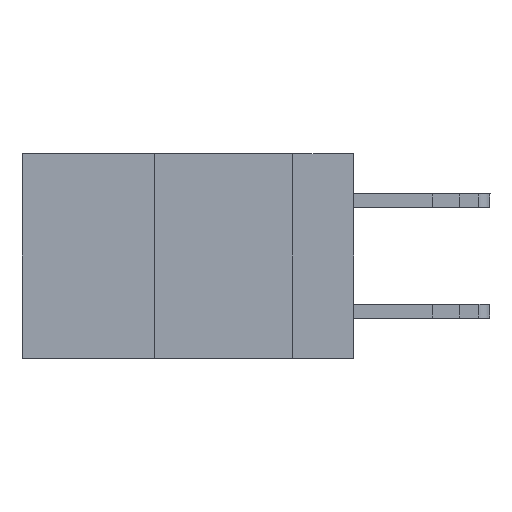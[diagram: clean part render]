
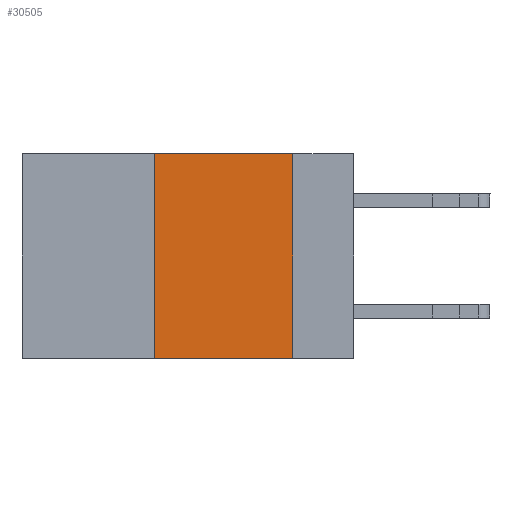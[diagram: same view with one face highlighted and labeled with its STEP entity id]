
A CAD part, left-side view. The second image highlights one B-rep face of the part: STEP entity #30505.
In plain terms, the highlighted planar face has unit normal (-1, 0, 0).
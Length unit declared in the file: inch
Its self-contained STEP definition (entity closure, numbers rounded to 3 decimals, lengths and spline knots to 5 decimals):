
#1029 = ORIENTED_EDGE ( 'NONE', *, *, #34617, .F. ) ;
#1294 = CARTESIAN_POINT ( 'NONE',  ( 0., 0.36, 0. ) ) ;
#1772 = EDGE_CURVE ( 'NONE', #18194, #14817, #13949, .T. ) ;
#2428 = CARTESIAN_POINT ( 'NONE',  ( 0., 0.36, 0. ) ) ;
#4544 = EDGE_CURVE ( 'NONE', #6720, #12037, #34415, .T. ) ;
#5986 = CARTESIAN_POINT ( 'NONE',  ( 0., 0.11, -0.37 ) ) ;
#6150 = CARTESIAN_POINT ( 'NONE',  ( 0., 0.6, 0. ) ) ;
#6337 = VECTOR ( 'NONE', #6770, 39.37008 ) ;
#6720 = VERTEX_POINT ( 'NONE', #1294 ) ;
#6770 = DIRECTION ( 'NONE',  ( 0., -1., 0. ) ) ;
#9180 = ORIENTED_EDGE ( 'NONE', *, *, #4544, .F. ) ;
#11246 = VECTOR ( 'NONE', #14752, 39.37008 ) ;
#11450 = DIRECTION ( 'NONE',  ( 0., 0., -1. ) ) ;
#11715 = ORIENTED_EDGE ( 'NONE', *, *, #1772, .T. ) ;
#11965 = EDGE_LOOP ( 'NONE', ( #1029, #9180, #12110, #11715 ) ) ;
#12037 = VERTEX_POINT ( 'NONE', #12791 ) ;
#12110 = ORIENTED_EDGE ( 'NONE', *, *, #13675, .F. ) ;
#12791 = CARTESIAN_POINT ( 'NONE',  ( 0., 0.11, 0. ) ) ;
#13675 = EDGE_CURVE ( 'NONE', #18194, #6720, #14356, .T. ) ;
#13949 = LINE ( 'NONE', #19732, #6337 ) ;
#14356 = LINE ( 'NONE', #2428, #24864 ) ;
#14752 = DIRECTION ( 'NONE',  ( 0., -1., 0. ) ) ;
#14792 = CARTESIAN_POINT ( 'NONE',  ( 0., 0.11, 0. ) ) ;
#14817 = VERTEX_POINT ( 'NONE', #5986 ) ;
#15346 = CARTESIAN_POINT ( 'NONE',  ( 0., 0.36, -0.37 ) ) ;
#17121 = VECTOR ( 'NONE', #28673, 39.37008 ) ;
#17985 = LINE ( 'NONE', #14792, #17121 ) ;
#18194 = VERTEX_POINT ( 'NONE', #15346 ) ;
#19430 = DIRECTION ( 'NONE',  ( 0., 0., 1. ) ) ;
#19732 = CARTESIAN_POINT ( 'NONE',  ( 0., 0.6, -0.37 ) ) ;
#20989 = FACE_OUTER_BOUND ( 'NONE', #11965, .T. ) ;
#24864 = VECTOR ( 'NONE', #19430, 39.37008 ) ;
#24945 = DIRECTION ( 'NONE',  ( 1., 0., 0. ) ) ;
#26743 = CARTESIAN_POINT ( 'NONE',  ( 0., 0.6, 0. ) ) ;
#28673 = DIRECTION ( 'NONE',  ( 0., 0., -1. ) ) ;
#29821 = PLANE ( 'NONE',  #31208 ) ;
#30505 = ADVANCED_FACE ( 'NONE', ( #20989 ), #29821, .F. ) ;
#31208 = AXIS2_PLACEMENT_3D ( 'NONE', #6150, #24945, #11450 ) ;
#34415 = LINE ( 'NONE', #26743, #11246 ) ;
#34617 = EDGE_CURVE ( 'NONE', #12037, #14817, #17985, .T. ) ;
